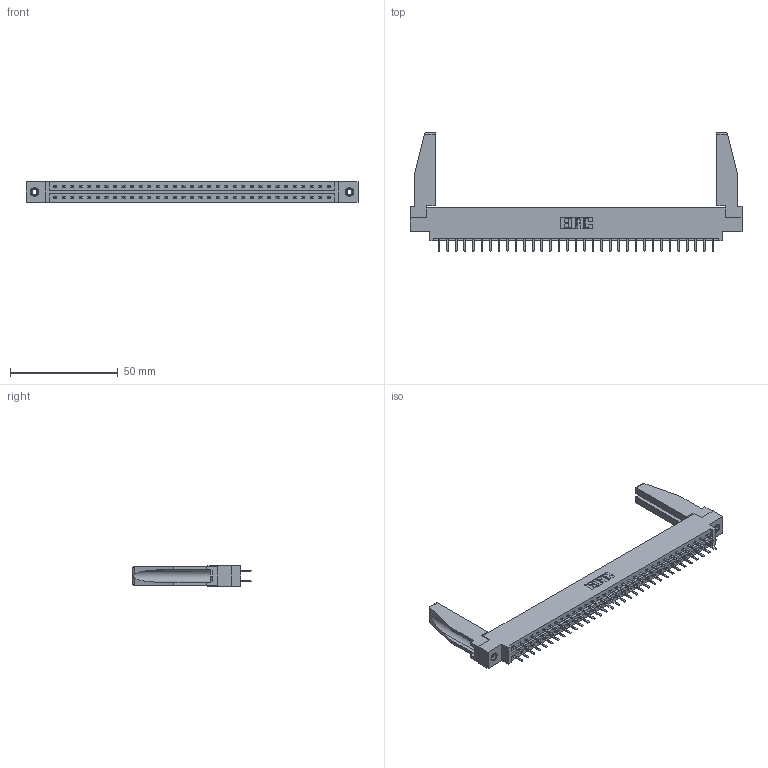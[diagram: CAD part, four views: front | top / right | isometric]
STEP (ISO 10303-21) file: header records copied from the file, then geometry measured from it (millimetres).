
FILE_DESCRIPTION (( 'STEP AP203' ), '1' );
FILE_NAME ('337-066-520-878.STEP', '2019-10-12T00:37:14', ( '' ), ( '' ), 'SwSTEP 2.0', 'SolidWorks 2016', '' );
FILE_SCHEMA (( 'CONFIG_CONTROL_DESIGN' ));
Length unit declared in the file: inch
Products named in the file (5): 307-220-078; 337-066-520-878; 345-292-001_345-293-120; 345-250-001_345-250-001-102; 337 Part_0.170 Offset - 0.156 Dia-TI
Assembly tree (71 placements, depth 2):
  337-066-520-878
    337 Part_0.170 Offset - 0.156 Dia-TI
    345-292-001_345-293-120  x66
    345-250-001_345-250-001-102  x2
    307-220-078  x2
Bounding box: 153.77 x 54.82 x 9.4 mm (x, y, z)
Volume: 19932.7 mm3; surface area: 21787.6 mm2
Topology: 71 solids, 71 shells, 4076 faces, 11807 edges, 7686 vertices
Faces by surface type: plane 2798, cylinder 1262, cone 12, torus 4
Entity records: 29436 total; most frequent: CARTESIAN_POINT 4980, ORIENTED_EDGE 4860, DIRECTION 4246, EDGE_CURVE 2430, VECTOR 2260, LINE 2260, VERTEX_POINT 1612, AXIS2_PLACEMENT_3D 993
